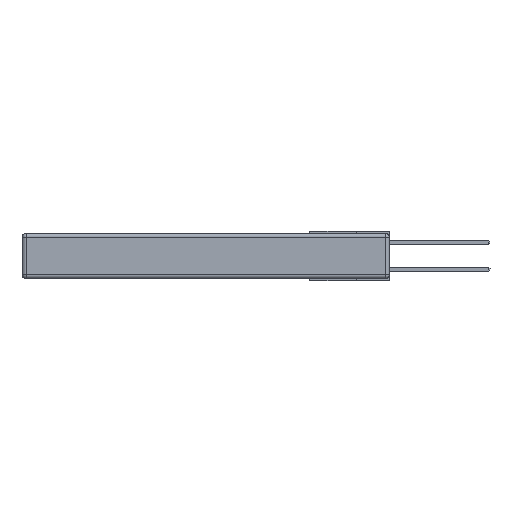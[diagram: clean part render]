
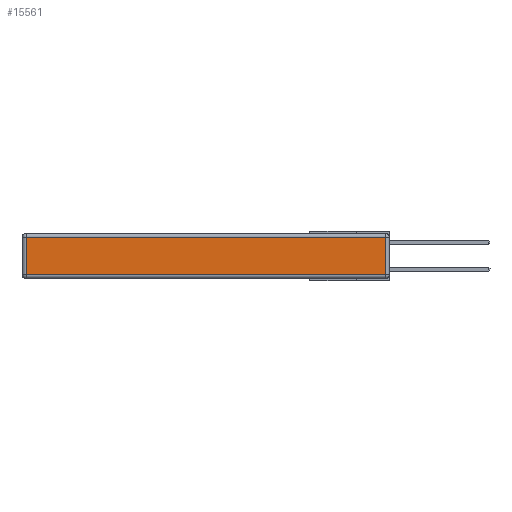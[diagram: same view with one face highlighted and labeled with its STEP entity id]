
A CAD part, left-side view. The second image highlights one B-rep face of the part: STEP entity #15561.
In plain terms, the highlighted planar face has unit normal (-1, 0, 0).
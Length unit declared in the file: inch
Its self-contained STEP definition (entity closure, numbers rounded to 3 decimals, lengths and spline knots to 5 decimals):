
#697 = VECTOR ( 'NONE', #24013, 39.37008 ) ;
#728 = VECTOR ( 'NONE', #8303, 39.37008 ) ;
#931 = CARTESIAN_POINT ( 'NONE',  ( 0., 0., -0.343 ) ) ;
#1052 = CARTESIAN_POINT ( 'NONE',  ( 0., 2.72, -0.343 ) ) ;
#1436 = FACE_OUTER_BOUND ( 'NONE', #2314, .T. ) ;
#1537 = DIRECTION ( 'NONE',  ( 0., 1., 0. ) ) ;
#2314 = EDGE_LOOP ( 'NONE', ( #4084, #14646, #8289, #22274 ) ) ;
#3362 = DIRECTION ( 'NONE',  ( 0., 0., 1. ) ) ;
#3965 = EDGE_CURVE ( 'NONE', #17840, #24125, #17480, .T. ) ;
#4084 = ORIENTED_EDGE ( 'NONE', *, *, #3965, .T. ) ;
#5605 = CARTESIAN_POINT ( 'NONE',  ( 0., 2.72, -0.313 ) ) ;
#8047 = DIRECTION ( 'NONE',  ( 0., -1., 0. ) ) ;
#8289 = ORIENTED_EDGE ( 'NONE', *, *, #19567, .T. ) ;
#8303 = DIRECTION ( 'NONE',  ( 0., 0., -1. ) ) ;
#8586 = CARTESIAN_POINT ( 'NONE',  ( 0., 0.03, -0.313 ) ) ;
#8672 = CARTESIAN_POINT ( 'NONE',  ( 0., 2.75, -0.03 ) ) ;
#13468 = LINE ( 'NONE', #14399, #697 ) ;
#14399 = CARTESIAN_POINT ( 'NONE',  ( 0., 0.03, -0.343 ) ) ;
#14646 = ORIENTED_EDGE ( 'NONE', *, *, #15328, .T. ) ;
#15328 = EDGE_CURVE ( 'NONE', #24125, #23181, #13468, .T. ) ;
#15357 = PLANE ( 'NONE',  #30672 ) ;
#15561 = ADVANCED_FACE ( 'NONE', ( #1436 ), #15357, .T. ) ;
#16020 = VERTEX_POINT ( 'NONE', #28764 ) ;
#16560 = LINE ( 'NONE', #8672, #25664 ) ;
#17480 = LINE ( 'NONE', #29708, #30782 ) ;
#17775 = DIRECTION ( 'NONE',  ( -1., 0., 0. ) ) ;
#17840 = VERTEX_POINT ( 'NONE', #5605 ) ;
#19567 = EDGE_CURVE ( 'NONE', #23181, #16020, #16560, .T. ) ;
#22274 = ORIENTED_EDGE ( 'NONE', *, *, #25087, .T. ) ;
#23181 = VERTEX_POINT ( 'NONE', #25433 ) ;
#23323 = LINE ( 'NONE', #1052, #728 ) ;
#24013 = DIRECTION ( 'NONE',  ( 0., 0., 1. ) ) ;
#24125 = VERTEX_POINT ( 'NONE', #8586 ) ;
#25087 = EDGE_CURVE ( 'NONE', #16020, #17840, #23323, .T. ) ;
#25433 = CARTESIAN_POINT ( 'NONE',  ( 0., 0.03, -0.03 ) ) ;
#25664 = VECTOR ( 'NONE', #1537, 39.37008 ) ;
#28764 = CARTESIAN_POINT ( 'NONE',  ( 0., 2.72, -0.03 ) ) ;
#29708 = CARTESIAN_POINT ( 'NONE',  ( 0., 0., -0.313 ) ) ;
#30672 = AXIS2_PLACEMENT_3D ( 'NONE', #931, #17775, #3362 ) ;
#30782 = VECTOR ( 'NONE', #8047, 39.37008 ) ;
